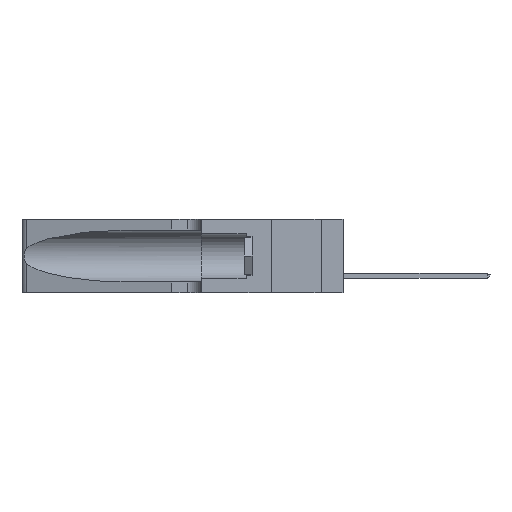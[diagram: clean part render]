
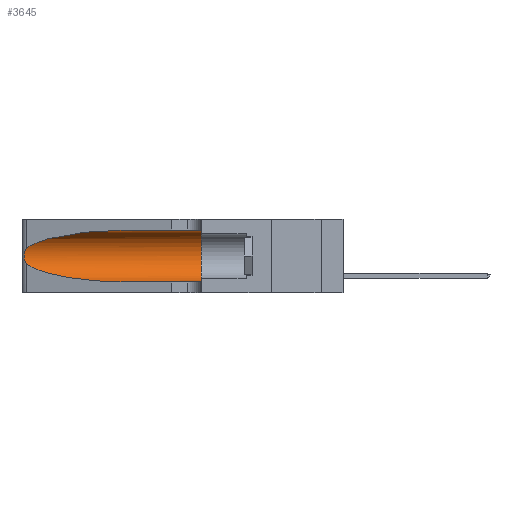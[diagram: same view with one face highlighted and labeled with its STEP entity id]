
A CAD part, left-side view. The second image highlights one B-rep face of the part: STEP entity #3645.
In plain terms, the highlighted cylindrical face has radius 3.308 mm (diameter 6.617 mm), a partial arc.
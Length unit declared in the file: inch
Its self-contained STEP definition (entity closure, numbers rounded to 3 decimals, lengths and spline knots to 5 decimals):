
#858 = EDGE_CURVE ( 'NONE', #22615, #23860, #8956, .T. ) ;
#1139 = CARTESIAN_POINT ( 'NONE',  ( 0.25487, 1.22718, 0.22369 ) ) ;
#1792 = EDGE_LOOP ( 'NONE', ( #15955, #22249, #9921, #3619, #2638, #13400 ) ) ;
#2189 = LINE ( 'NONE', #3685, #2835 ) ;
#2638 = ORIENTED_EDGE ( 'NONE', *, *, #5880, .F. ) ;
#2835 = VECTOR ( 'NONE', #13800, 39.37008 ) ;
#3311 = AXIS2_PLACEMENT_3D ( 'NONE', #10939, #17091, #25371 ) ;
#3367 = FACE_OUTER_BOUND ( 'NONE', #1792, .T. ) ;
#3520 = CARTESIAN_POINT ( 'NONE',  ( 0.1305, 1.61858, 0.31525 ) ) ;
#3619 = ORIENTED_EDGE ( 'NONE', *, *, #17937, .T. ) ;
#3645 = ADVANCED_FACE ( 'NONE', ( #3367 ), #18410, .F. ) ;
#3671 = CARTESIAN_POINT ( 'NONE',  ( 0.25487, 1.22718, 0.14631 ) ) ;
#3685 = CARTESIAN_POINT ( 'NONE',  ( 0.1305, 1.61858, 0.05475 ) ) ;
#4191 = CARTESIAN_POINT ( 'NONE',  ( 0.25555, 1.22994, 0.2215 ) ) ;
#4798 = VERTEX_POINT ( 'NONE', #3671 ) ;
#5069 = CARTESIAN_POINT ( 'NONE',  ( 0.25487, 1.22718, 0.14631 ) ) ;
#5565 = B_SPLINE_CURVE_WITH_KNOTS ( 'NONE', 3,
 ( #24443, #4191, #20503, #6119, #14474, #20584, #12089, #20420, #10205, #18512, #16270, #7962, #8211, #24611 ),
 .UNSPECIFIED., .F., .F.,
 ( 4, 2, 2, 2, 2, 2, 4 ),
 ( 0., 0.00027, 0.00053, 0.00107, 0.0016, 0.00187, 0.00214 ),
 .UNSPECIFIED. ) ;
#5601 = LINE ( 'NONE', #3520, #8415 ) ;
#5880 = EDGE_CURVE ( 'NONE', #20871, #13419, #16071, .T. ) ;
#6119 = CARTESIAN_POINT ( 'NONE',  ( 0.25787, 1.23484, 0.2124 ) ) ;
#7036 = CARTESIAN_POINT ( 'NONE',  ( 0.18966, 0.96281, 0.05475 ) ) ;
#7962 = CARTESIAN_POINT ( 'NONE',  ( 0.25639, 1.23186, 0.15144 ) ) ;
#8211 = CARTESIAN_POINT ( 'NONE',  ( 0.25555, 1.22993, 0.14849 ) ) ;
#8415 = VECTOR ( 'NONE', #26452, 39.37008 ) ;
#8956 =( BOUNDED_CURVE ( )  B_SPLINE_CURVE ( 3, ( #19353, #23937, #17458, #22505 ),
 .UNSPECIFIED., .F., .F. ) 
 B_SPLINE_CURVE_WITH_KNOTS ( ( 4, 4 ),
 ( 1.5708, 2.84003 ),
 .UNSPECIFIED. ) 
 CURVE ( )  GEOMETRIC_REPRESENTATION_ITEM ( )  RATIONAL_B_SPLINE_CURVE ( ( 1., 0.87, 0.87, 1. ) ) 
 REPRESENTATION_ITEM ( '' )  );
#9921 = ORIENTED_EDGE ( 'NONE', *, *, #12742, .T. ) ;
#9992 = EDGE_CURVE ( 'NONE', #22615, #20871, #5601, .T. ) ;
#10124 = DIRECTION ( 'NONE',  ( 0., -1., 0. ) ) ;
#10205 = CARTESIAN_POINT ( 'NONE',  ( 0.26017, 1.23833, 0.17102 ) ) ;
#10939 = CARTESIAN_POINT ( 'NONE',  ( 0.1305, 0.35, 0.185 ) ) ;
#12085 = CARTESIAN_POINT ( 'NONE',  ( 0.1305, 1.61858, 0.185 ) ) ;
#12089 = CARTESIAN_POINT ( 'NONE',  ( 0.26075, 1.23896, 0.19203 ) ) ;
#12152 = AXIS2_PLACEMENT_3D ( 'NONE', #12085, #10124, #18167 ) ;
#12742 = EDGE_CURVE ( 'NONE', #4798, #17168, #15014, .T. ) ;
#12950 = CARTESIAN_POINT ( 'NONE',  ( 0.1305, 0.72297, 0.05475 ) ) ;
#13191 = CARTESIAN_POINT ( 'NONE',  ( 0.1305, 0.72297, 0.05475 ) ) ;
#13400 = ORIENTED_EDGE ( 'NONE', *, *, #9992, .F. ) ;
#13419 = VERTEX_POINT ( 'NONE', #19186 ) ;
#13800 = DIRECTION ( 'NONE',  ( 0., -1., 0. ) ) ;
#14474 = CARTESIAN_POINT ( 'NONE',  ( 0.25854, 1.2359, 0.20912 ) ) ;
#14735 = CARTESIAN_POINT ( 'NONE',  ( 0.1305, 0.72297, 0.31525 ) ) ;
#15014 =( BOUNDED_CURVE ( )  B_SPLINE_CURVE ( 3, ( #5069, #21340, #7036, #13191 ),
 .UNSPECIFIED., .F., .F. ) 
 B_SPLINE_CURVE_WITH_KNOTS ( ( 4, 4 ),
 ( 3.44316, 4.71239 ),
 .UNSPECIFIED. ) 
 CURVE ( )  GEOMETRIC_REPRESENTATION_ITEM ( )  RATIONAL_B_SPLINE_CURVE ( ( 1., 0.87, 0.87, 1. ) ) 
 REPRESENTATION_ITEM ( '' )  );
#15955 = ORIENTED_EDGE ( 'NONE', *, *, #858, .T. ) ;
#16071 = CIRCLE ( 'NONE', #3311, 0.13025 ) ;
#16270 = CARTESIAN_POINT ( 'NONE',  ( 0.25789, 1.23486, 0.15765 ) ) ;
#17091 = DIRECTION ( 'NONE',  ( 0., 1., 0. ) ) ;
#17168 = VERTEX_POINT ( 'NONE', #12950 ) ;
#17458 = CARTESIAN_POINT ( 'NONE',  ( 0.2373, 1.15595, 0.28018 ) ) ;
#17937 = EDGE_CURVE ( 'NONE', #17168, #13419, #2189, .T. ) ;
#18167 = DIRECTION ( 'NONE',  ( 0., 0., -1. ) ) ;
#18410 = CYLINDRICAL_SURFACE ( 'NONE', #12152, 0.13025 ) ;
#18509 = EDGE_CURVE ( 'NONE', #23860, #4798, #5565, .T. ) ;
#18512 = CARTESIAN_POINT ( 'NONE',  ( 0.25856, 1.23593, 0.16098 ) ) ;
#19186 = CARTESIAN_POINT ( 'NONE',  ( 0.1305, 0.35, 0.05475 ) ) ;
#19353 = CARTESIAN_POINT ( 'NONE',  ( 0.1305, 0.72297, 0.31525 ) ) ;
#20029 = CARTESIAN_POINT ( 'NONE',  ( 0.1305, 0.35, 0.31525 ) ) ;
#20420 = CARTESIAN_POINT ( 'NONE',  ( 0.26075, 1.23896, 0.178 ) ) ;
#20503 = CARTESIAN_POINT ( 'NONE',  ( 0.25639, 1.23184, 0.21858 ) ) ;
#20584 = CARTESIAN_POINT ( 'NONE',  ( 0.26018, 1.23835, 0.19895 ) ) ;
#20871 = VERTEX_POINT ( 'NONE', #20029 ) ;
#21340 = CARTESIAN_POINT ( 'NONE',  ( 0.2373, 1.15595, 0.08982 ) ) ;
#22249 = ORIENTED_EDGE ( 'NONE', *, *, #18509, .T. ) ;
#22505 = CARTESIAN_POINT ( 'NONE',  ( 0.25487, 1.22718, 0.22369 ) ) ;
#22615 = VERTEX_POINT ( 'NONE', #14735 ) ;
#23860 = VERTEX_POINT ( 'NONE', #1139 ) ;
#23937 = CARTESIAN_POINT ( 'NONE',  ( 0.18966, 0.96281, 0.31525 ) ) ;
#24443 = CARTESIAN_POINT ( 'NONE',  ( 0.25487, 1.22718, 0.22369 ) ) ;
#24611 = CARTESIAN_POINT ( 'NONE',  ( 0.25487, 1.22718, 0.14631 ) ) ;
#25371 = DIRECTION ( 'NONE',  ( 0., 0., 1. ) ) ;
#26452 = DIRECTION ( 'NONE',  ( 0., -1., 0. ) ) ;
